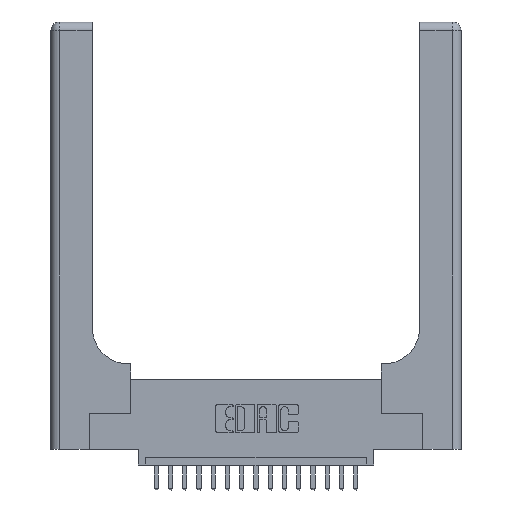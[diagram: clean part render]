
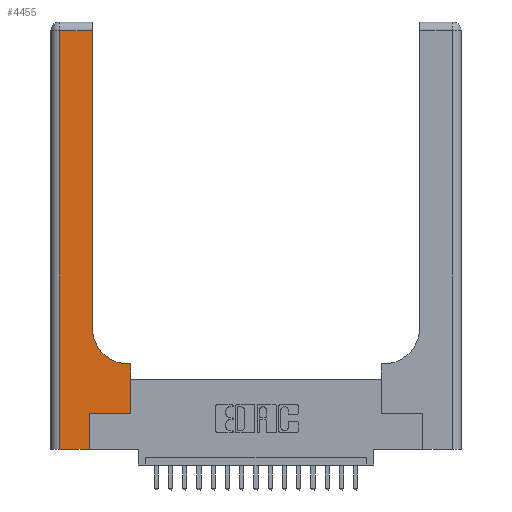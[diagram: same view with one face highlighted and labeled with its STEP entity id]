
A CAD part, top view. The second image highlights one B-rep face of the part: STEP entity #4455.
In plain terms, the highlighted planar face has unit normal (0, 0, 1).
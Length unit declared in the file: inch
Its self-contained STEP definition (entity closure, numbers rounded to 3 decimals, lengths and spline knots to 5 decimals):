
#3 = ORIENTED_EDGE ( 'NONE', *, *, #9239, .T. ) ;
#423 = ORIENTED_EDGE ( 'NONE', *, *, #9521, .T. ) ;
#624 = VERTEX_POINT ( 'NONE', #827 ) ;
#708 = VECTOR ( 'NONE', #5180, 39.37008 ) ;
#827 = CARTESIAN_POINT ( 'NONE',  ( 0.5415, 0.6, 0.37 ) ) ;
#1177 = CIRCLE ( 'NONE', #15849, 0.25 ) ;
#1188 = LINE ( 'NONE', #14583, #708 ) ;
#1359 = VERTEX_POINT ( 'NONE', #16515 ) ;
#1468 = VECTOR ( 'NONE', #9787, 39.37008 ) ;
#2186 = CARTESIAN_POINT ( 'NONE',  ( 0., 0., 0.37 ) ) ;
#2633 = EDGE_CURVE ( 'NONE', #18206, #14372, #10896, .T. ) ;
#2830 = LINE ( 'NONE', #14784, #12247 ) ;
#2935 = VECTOR ( 'NONE', #10495, 39.37008 ) ;
#3023 = VERTEX_POINT ( 'NONE', #6071 ) ;
#3043 = ORIENTED_EDGE ( 'NONE', *, *, #15510, .T. ) ;
#3128 = CARTESIAN_POINT ( 'NONE',  ( 0.269, 0.25, 0.37 ) ) ;
#3268 = ORIENTED_EDGE ( 'NONE', *, *, #5575, .T. ) ;
#3631 = CARTESIAN_POINT ( 'NONE',  ( 0.2915, 3., 0.37 ) ) ;
#3878 = CARTESIAN_POINT ( 'NONE',  ( 0.269, 0., 0.37 ) ) ;
#4164 = ORIENTED_EDGE ( 'NONE', *, *, #13053, .T. ) ;
#4325 = EDGE_CURVE ( 'NONE', #7835, #1359, #1188, .T. ) ;
#4455 = ADVANCED_FACE ( 'NONE', ( #15030 ), #10424, .F. ) ;
#5180 = DIRECTION ( 'NONE',  ( -1., 0., 0. ) ) ;
#5575 = EDGE_CURVE ( 'NONE', #3023, #624, #2830, .T. ) ;
#5636 = LINE ( 'NONE', #3878, #11538 ) ;
#5740 = CARTESIAN_POINT ( 'NONE',  ( 0., 3., 0.37 ) ) ;
#5846 = ORIENTED_EDGE ( 'NONE', *, *, #4325, .T. ) ;
#5910 = LINE ( 'NONE', #3631, #1468 ) ;
#6071 = CARTESIAN_POINT ( 'NONE',  ( 0.5585, 0.6, 0.37 ) ) ;
#6482 = DIRECTION ( 'NONE',  ( 1., 0., 0. ) ) ;
#7835 = VERTEX_POINT ( 'NONE', #19584 ) ;
#7877 = VERTEX_POINT ( 'NONE', #11867 ) ;
#7971 = LINE ( 'NONE', #11620, #19995 ) ;
#8523 = DIRECTION ( 'NONE',  ( 0., 1., 0. ) ) ;
#8592 = CARTESIAN_POINT ( 'NONE',  ( 0.269, 0., 0.37 ) ) ;
#8701 = DIRECTION ( 'NONE',  ( 1., 0., 0. ) ) ;
#9171 = LINE ( 'NONE', #11316, #2935 ) ;
#9212 = CARTESIAN_POINT ( 'NONE',  ( 0.06, 0., 0.37 ) ) ;
#9239 = EDGE_CURVE ( 'NONE', #1359, #9332, #9171, .T. ) ;
#9332 = VERTEX_POINT ( 'NONE', #9212 ) ;
#9521 = EDGE_CURVE ( 'NONE', #7877, #7835, #5910, .T. ) ;
#9787 = DIRECTION ( 'NONE',  ( 0., 1., 0. ) ) ;
#9842 = EDGE_CURVE ( 'NONE', #9332, #11428, #18937, .T. ) ;
#10424 = PLANE ( 'NONE',  #12506 ) ;
#10495 = DIRECTION ( 'NONE',  ( 0., -1., 0. ) ) ;
#10896 = LINE ( 'NONE', #3128, #16798 ) ;
#11316 = CARTESIAN_POINT ( 'NONE',  ( 0.06, 3., 0.37 ) ) ;
#11404 = DIRECTION ( 'NONE',  ( 0., 0., -1. ) ) ;
#11428 = VERTEX_POINT ( 'NONE', #8592 ) ;
#11538 = VECTOR ( 'NONE', #8523, 39.37008 ) ;
#11620 = CARTESIAN_POINT ( 'NONE',  ( 0.5585, 0.25, 0.37 ) ) ;
#11867 = CARTESIAN_POINT ( 'NONE',  ( 0.2915, 0.85, 0.37 ) ) ;
#12247 = VECTOR ( 'NONE', #19485, 39.37008 ) ;
#12506 = AXIS2_PLACEMENT_3D ( 'NONE', #5740, #19589, #19826 ) ;
#13053 = EDGE_CURVE ( 'NONE', #14372, #3023, #7971, .T. ) ;
#13654 = ORIENTED_EDGE ( 'NONE', *, *, #15472, .T. ) ;
#13984 = ORIENTED_EDGE ( 'NONE', *, *, #9842, .T. ) ;
#14062 = VECTOR ( 'NONE', #8701, 39.37008 ) ;
#14372 = VERTEX_POINT ( 'NONE', #15636 ) ;
#14583 = CARTESIAN_POINT ( 'NONE',  ( 0., 2.94, 0.37 ) ) ;
#14628 = DIRECTION ( 'NONE',  ( 1., 0., 0. ) ) ;
#14784 = CARTESIAN_POINT ( 'NONE',  ( 0.2915, 0.6, 0.37 ) ) ;
#15029 = DIRECTION ( 'NONE',  ( 0., 1., 0. ) ) ;
#15030 = FACE_OUTER_BOUND ( 'NONE', #16295, .T. ) ;
#15472 = EDGE_CURVE ( 'NONE', #624, #7877, #1177, .T. ) ;
#15510 = EDGE_CURVE ( 'NONE', #11428, #18206, #5636, .T. ) ;
#15636 = CARTESIAN_POINT ( 'NONE',  ( 0.5585, 0.25, 0.37 ) ) ;
#15849 = AXIS2_PLACEMENT_3D ( 'NONE', #19445, #11404, #14628 ) ;
#16295 = EDGE_LOOP ( 'NONE', ( #423, #5846, #3, #13984, #3043, #18257, #4164, #3268, #13654 ) ) ;
#16515 = CARTESIAN_POINT ( 'NONE',  ( 0.06, 2.94, 0.37 ) ) ;
#16798 = VECTOR ( 'NONE', #6482, 39.37008 ) ;
#18206 = VERTEX_POINT ( 'NONE', #20042 ) ;
#18257 = ORIENTED_EDGE ( 'NONE', *, *, #2633, .T. ) ;
#18937 = LINE ( 'NONE', #2186, #14062 ) ;
#19445 = CARTESIAN_POINT ( 'NONE',  ( 0.5415, 0.85, 0.37 ) ) ;
#19485 = DIRECTION ( 'NONE',  ( -1., 0., 0. ) ) ;
#19584 = CARTESIAN_POINT ( 'NONE',  ( 0.2915, 2.94, 0.37 ) ) ;
#19589 = DIRECTION ( 'NONE',  ( 0., 0., -1. ) ) ;
#19826 = DIRECTION ( 'NONE',  ( -1., 0., 0. ) ) ;
#19995 = VECTOR ( 'NONE', #15029, 39.37008 ) ;
#20042 = CARTESIAN_POINT ( 'NONE',  ( 0.269, 0.25, 0.37 ) ) ;
